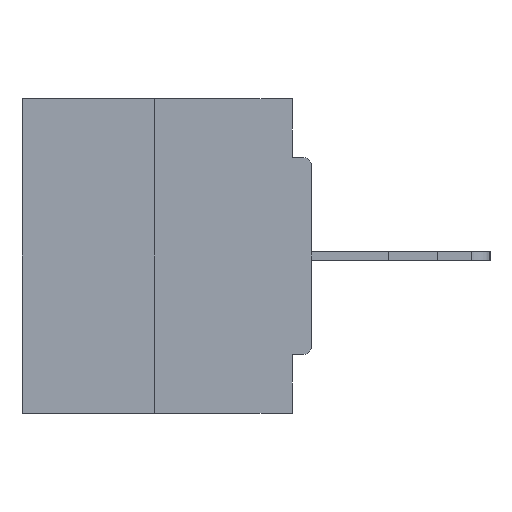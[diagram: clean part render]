
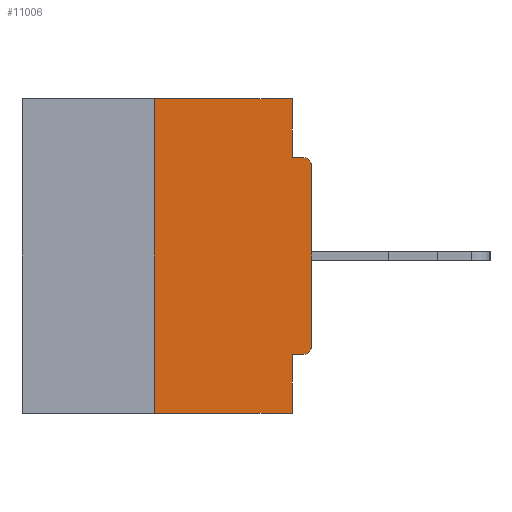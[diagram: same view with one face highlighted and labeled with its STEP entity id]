
A CAD part, left-side view. The second image highlights one B-rep face of the part: STEP entity #11006.
In plain terms, the highlighted planar face has unit normal (-1, 0, 0).
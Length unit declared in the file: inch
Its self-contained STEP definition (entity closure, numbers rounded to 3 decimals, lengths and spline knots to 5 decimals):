
#671 = EDGE_CURVE ( 'NONE', #20046, #10777, #13451, .T. ) ;
#819 = VERTEX_POINT ( 'NONE', #12128 ) ;
#908 = VERTEX_POINT ( 'NONE', #29132 ) ;
#1266 = VECTOR ( 'NONE', #2975, 39.37008 ) ;
#1443 = CIRCLE ( 'NONE', #4016, 0.015 ) ;
#1454 = EDGE_LOOP ( 'NONE', ( #2590, #5305, #8745, #13167, #7158, #16081, #29001, #17848, #1827, #12614 ) ) ;
#1779 = LINE ( 'NONE', #23930, #25535 ) ;
#1827 = ORIENTED_EDGE ( 'NONE', *, *, #15511, .F. ) ;
#1942 = DIRECTION ( 'NONE',  ( 0., 0., -1. ) ) ;
#2443 = CARTESIAN_POINT ( 'NONE',  ( 0., 0.031, -0.5 ) ) ;
#2590 = ORIENTED_EDGE ( 'NONE', *, *, #671, .F. ) ;
#2975 = DIRECTION ( 'NONE',  ( 0., -1., 0. ) ) ;
#3077 = CIRCLE ( 'NONE', #29208, 0.015 ) ;
#3341 = VERTEX_POINT ( 'NONE', #19229 ) ;
#4016 = AXIS2_PLACEMENT_3D ( 'NONE', #16204, #5937, #23432 ) ;
#4082 = EDGE_CURVE ( 'NONE', #10777, #7342, #1779, .T. ) ;
#4258 = CARTESIAN_POINT ( 'NONE',  ( 0., 0.46, 0. ) ) ;
#4465 = EDGE_CURVE ( 'NONE', #819, #20265, #9612, .T. ) ;
#5213 = CARTESIAN_POINT ( 'NONE',  ( 0., 0., -0.0935 ) ) ;
#5305 = ORIENTED_EDGE ( 'NONE', *, *, #10031, .F. ) ;
#5816 = DIRECTION ( 'NONE',  ( 0., -1., 0. ) ) ;
#5937 = DIRECTION ( 'NONE',  ( -1., 0., 0. ) ) ;
#7031 = DIRECTION ( 'NONE',  ( 0., 0., 1. ) ) ;
#7158 = ORIENTED_EDGE ( 'NONE', *, *, #24748, .F. ) ;
#7245 = DIRECTION ( 'NONE',  ( 0., 0., -1. ) ) ;
#7285 = CARTESIAN_POINT ( 'NONE',  ( 0., 0.25, -0.5 ) ) ;
#7342 = VERTEX_POINT ( 'NONE', #25803 ) ;
#7967 = CARTESIAN_POINT ( 'NONE',  ( 0., 0., -0.1085 ) ) ;
#8379 = PLANE ( 'NONE',  #12475 ) ;
#8745 = ORIENTED_EDGE ( 'NONE', *, *, #11700, .T. ) ;
#9523 = CARTESIAN_POINT ( 'NONE',  ( 0., 0.015, -0.3915 ) ) ;
#9612 = LINE ( 'NONE', #28553, #11835 ) ;
#10031 = EDGE_CURVE ( 'NONE', #15779, #20046, #13944, .T. ) ;
#10464 = VECTOR ( 'NONE', #25035, 39.37008 ) ;
#10777 = VERTEX_POINT ( 'NONE', #21568 ) ;
#11006 = ADVANCED_FACE ( 'NONE', ( #12891 ), #8379, .F. ) ;
#11700 = EDGE_CURVE ( 'NONE', #15779, #26194, #30217, .T. ) ;
#11835 = VECTOR ( 'NONE', #16667, 39.37008 ) ;
#12128 = CARTESIAN_POINT ( 'NONE',  ( 0., 0., -0.3915 ) ) ;
#12475 = AXIS2_PLACEMENT_3D ( 'NONE', #25242, #15305, #18175 ) ;
#12614 = ORIENTED_EDGE ( 'NONE', *, *, #4082, .F. ) ;
#12891 = FACE_OUTER_BOUND ( 'NONE', #1454, .T. ) ;
#12918 = LINE ( 'NONE', #5213, #1266 ) ;
#13167 = ORIENTED_EDGE ( 'NONE', *, *, #13840, .F. ) ;
#13451 = LINE ( 'NONE', #4258, #26761 ) ;
#13840 = EDGE_CURVE ( 'NONE', #3341, #26194, #27130, .T. ) ;
#13944 = LINE ( 'NONE', #29042, #23667 ) ;
#14391 = LINE ( 'NONE', #31536, #25183 ) ;
#15305 = DIRECTION ( 'NONE',  ( 1., 0., 0. ) ) ;
#15511 = EDGE_CURVE ( 'NONE', #7342, #908, #12918, .T. ) ;
#15779 = VERTEX_POINT ( 'NONE', #7285 ) ;
#16081 = ORIENTED_EDGE ( 'NONE', *, *, #29336, .T. ) ;
#16204 = CARTESIAN_POINT ( 'NONE',  ( 0., 0.015, -0.1085 ) ) ;
#16667 = DIRECTION ( 'NONE',  ( 0., 0., 1. ) ) ;
#17043 = DIRECTION ( 'NONE',  ( -1., 0., 0. ) ) ;
#17848 = ORIENTED_EDGE ( 'NONE', *, *, #19308, .T. ) ;
#18175 = DIRECTION ( 'NONE',  ( 0., 0., -1. ) ) ;
#18183 = CARTESIAN_POINT ( 'NONE',  ( 0., 0.46, -0.5 ) ) ;
#18605 = VECTOR ( 'NONE', #5816, 39.37008 ) ;
#19229 = CARTESIAN_POINT ( 'NONE',  ( 0., 0.031, -0.4065 ) ) ;
#19308 = EDGE_CURVE ( 'NONE', #20265, #908, #1443, .T. ) ;
#20046 = VERTEX_POINT ( 'NONE', #28386 ) ;
#20265 = VERTEX_POINT ( 'NONE', #7967 ) ;
#21568 = CARTESIAN_POINT ( 'NONE',  ( 0., 0.031, 0. ) ) ;
#21609 = DIRECTION ( 'NONE',  ( 0., 1., 0. ) ) ;
#21980 = CARTESIAN_POINT ( 'NONE',  ( 0., 0.031, -0.5 ) ) ;
#23243 = DIRECTION ( 'NONE',  ( 0., -1., 0. ) ) ;
#23432 = DIRECTION ( 'NONE',  ( 0., 0., -1. ) ) ;
#23641 = VERTEX_POINT ( 'NONE', #27970 ) ;
#23667 = VECTOR ( 'NONE', #7031, 39.37008 ) ;
#23930 = CARTESIAN_POINT ( 'NONE',  ( 0., 0.031, 0. ) ) ;
#24748 = EDGE_CURVE ( 'NONE', #23641, #3341, #14391, .T. ) ;
#25035 = DIRECTION ( 'NONE',  ( 0., 0., -1. ) ) ;
#25183 = VECTOR ( 'NONE', #21609, 39.37008 ) ;
#25242 = CARTESIAN_POINT ( 'NONE',  ( 0., 0.46, 0. ) ) ;
#25535 = VECTOR ( 'NONE', #1942, 39.37008 ) ;
#25803 = CARTESIAN_POINT ( 'NONE',  ( 0., 0.031, -0.0935 ) ) ;
#26194 = VERTEX_POINT ( 'NONE', #2443 ) ;
#26761 = VECTOR ( 'NONE', #23243, 39.37008 ) ;
#27130 = LINE ( 'NONE', #21980, #10464 ) ;
#27970 = CARTESIAN_POINT ( 'NONE',  ( 0., 0.015, -0.4065 ) ) ;
#28386 = CARTESIAN_POINT ( 'NONE',  ( 0., 0.25, 0. ) ) ;
#28553 = CARTESIAN_POINT ( 'NONE',  ( 0., 0., 0. ) ) ;
#29001 = ORIENTED_EDGE ( 'NONE', *, *, #4465, .T. ) ;
#29042 = CARTESIAN_POINT ( 'NONE',  ( 0., 0.25, 0. ) ) ;
#29132 = CARTESIAN_POINT ( 'NONE',  ( 0., 0.015, -0.0935 ) ) ;
#29208 = AXIS2_PLACEMENT_3D ( 'NONE', #9523, #17043, #7245 ) ;
#29336 = EDGE_CURVE ( 'NONE', #23641, #819, #3077, .T. ) ;
#30217 = LINE ( 'NONE', #18183, #18605 ) ;
#31536 = CARTESIAN_POINT ( 'NONE',  ( 0., 0., -0.4065 ) ) ;
